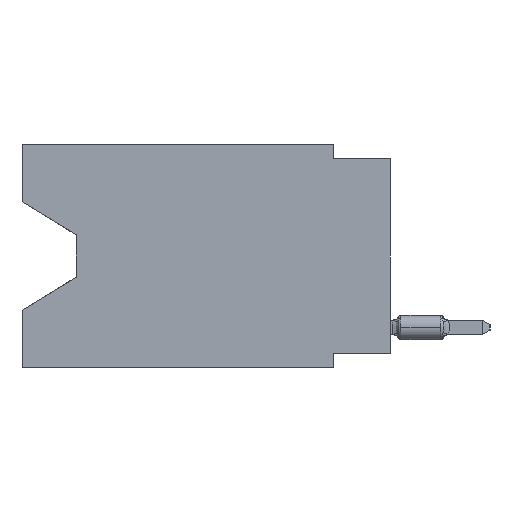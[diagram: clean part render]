
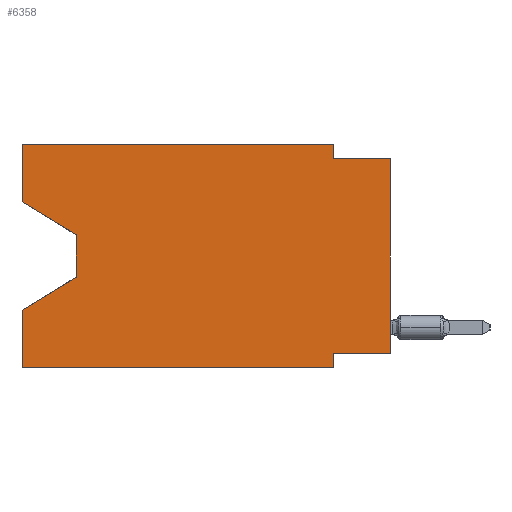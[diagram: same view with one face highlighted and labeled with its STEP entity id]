
A CAD part, left-side view. The second image highlights one B-rep face of the part: STEP entity #6358.
In plain terms, the highlighted planar face has unit normal (-1, 0, 0).
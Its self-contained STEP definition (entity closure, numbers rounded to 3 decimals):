
#1512 = VECTOR ( 'NONE', #14269, 1000. ) ;
#1819 = VERTEX_POINT ( 'NONE', #41051 ) ;
#2032 = EDGE_CURVE ( 'NONE', #39191, #20575, #32873, .T. ) ;
#2313 = LINE ( 'NONE', #47845, #11369 ) ;
#2354 = EDGE_CURVE ( 'NONE', #15973, #26219, #27699, .T. ) ;
#2417 = CARTESIAN_POINT ( 'NONE',  ( 0., 13.97, -4.013 ) ) ;
#2497 = DIRECTION ( 'NONE',  ( 0., 0., -1. ) ) ;
#3361 = EDGE_LOOP ( 'NONE', ( #6334, #10303, #36946, #3915, #14482, #22996, #16366, #15997, #44601, #26552, #22418, #24889 ) ) ;
#3915 = ORIENTED_EDGE ( 'NONE', *, *, #47639, .F. ) ;
#3995 = EDGE_CURVE ( 'NONE', #39756, #20575, #34410, .T. ) ;
#4462 = CARTESIAN_POINT ( 'NONE',  ( 0., 2.54, 0. ) ) ;
#6122 = EDGE_CURVE ( 'NONE', #18912, #26900, #34582, .T. ) ;
#6334 = ORIENTED_EDGE ( 'NONE', *, *, #33311, .T. ) ;
#6358 = ADVANCED_FACE ( 'NONE', ( #40655 ), #7126, .F. ) ;
#6839 = CARTESIAN_POINT ( 'NONE',  ( 0., 13.97, -5.893 ) ) ;
#6944 = CARTESIAN_POINT ( 'NONE',  ( 0., 0., -0.635 ) ) ;
#6964 = DIRECTION ( 'NONE',  ( 0., 0., 1. ) ) ;
#7126 = PLANE ( 'NONE',  #29096 ) ;
#7190 = LINE ( 'NONE', #6944, #41994 ) ;
#7594 = VERTEX_POINT ( 'NONE', #29432 ) ;
#10260 = EDGE_CURVE ( 'NONE', #26900, #7594, #7190, .T. ) ;
#10303 = ORIENTED_EDGE ( 'NONE', *, *, #11904, .T. ) ;
#10648 = LINE ( 'NONE', #25588, #21069 ) ;
#11043 = DIRECTION ( 'NONE',  ( 1., 0., 0. ) ) ;
#11065 = CARTESIAN_POINT ( 'NONE',  ( 0., 2.54, -0.635 ) ) ;
#11369 = VECTOR ( 'NONE', #31947, 1000. ) ;
#11904 = EDGE_CURVE ( 'NONE', #18382, #1819, #29109, .T. ) ;
#12140 = CARTESIAN_POINT ( 'NONE',  ( 0., 2.54, -9.906 ) ) ;
#12975 = DIRECTION ( 'NONE',  ( 0., 0., 1. ) ) ;
#12997 = DIRECTION ( 'NONE',  ( 0., 0., 1. ) ) ;
#13322 = DIRECTION ( 'NONE',  ( 0., -1., 0. ) ) ;
#13789 = CARTESIAN_POINT ( 'NONE',  ( 0., 13.97, -4.013 ) ) ;
#13973 = EDGE_CURVE ( 'NONE', #30000, #7594, #10648, .T. ) ;
#14126 = CARTESIAN_POINT ( 'NONE',  ( 0., 16.383, -2.546 ) ) ;
#14269 = DIRECTION ( 'NONE',  ( 0., -1., 0. ) ) ;
#14366 = DIRECTION ( 'NONE',  ( 0., -0.855, -0.519 ) ) ;
#14482 = ORIENTED_EDGE ( 'NONE', *, *, #2032, .T. ) ;
#14748 = VERTEX_POINT ( 'NONE', #17641 ) ;
#15544 = VECTOR ( 'NONE', #16872, 1000. ) ;
#15973 = VERTEX_POINT ( 'NONE', #34467 ) ;
#15997 = ORIENTED_EDGE ( 'NONE', *, *, #13973, .T. ) ;
#16366 = ORIENTED_EDGE ( 'NONE', *, *, #46910, .F. ) ;
#16872 = DIRECTION ( 'NONE',  ( 0., 0., -1. ) ) ;
#17641 = CARTESIAN_POINT ( 'NONE',  ( 0., 16.383, -7.36 ) ) ;
#18382 = VERTEX_POINT ( 'NONE', #13789 ) ;
#18912 = VERTEX_POINT ( 'NONE', #19013 ) ;
#19013 = CARTESIAN_POINT ( 'NONE',  ( 0., 2.54, 0. ) ) ;
#20175 = CARTESIAN_POINT ( 'NONE',  ( 0., 16.383, 0. ) ) ;
#20575 = VERTEX_POINT ( 'NONE', #33538 ) ;
#21069 = VECTOR ( 'NONE', #6964, 1000. ) ;
#21534 = LINE ( 'NONE', #6839, #48112 ) ;
#21873 = DIRECTION ( 'NONE',  ( 0., -1., 0. ) ) ;
#22011 = DIRECTION ( 'NONE',  ( 0., 0.855, -0.519 ) ) ;
#22083 = CARTESIAN_POINT ( 'NONE',  ( 0., 16.383, -9.906 ) ) ;
#22418 = ORIENTED_EDGE ( 'NONE', *, *, #43143, .F. ) ;
#22996 = ORIENTED_EDGE ( 'NONE', *, *, #3995, .F. ) ;
#23609 = LINE ( 'NONE', #20175, #24547 ) ;
#24547 = VECTOR ( 'NONE', #13322, 1000. ) ;
#24553 = VECTOR ( 'NONE', #14366, 1000. ) ;
#24889 = ORIENTED_EDGE ( 'NONE', *, *, #2354, .F. ) ;
#25588 = CARTESIAN_POINT ( 'NONE',  ( 0., 0., 0. ) ) ;
#26219 = VERTEX_POINT ( 'NONE', #42239 ) ;
#26552 = ORIENTED_EDGE ( 'NONE', *, *, #6122, .F. ) ;
#26900 = VERTEX_POINT ( 'NONE', #11065 ) ;
#27699 = LINE ( 'NONE', #42617, #42175 ) ;
#28408 = CARTESIAN_POINT ( 'NONE',  ( 0., 16.383, 0. ) ) ;
#29096 = AXIS2_PLACEMENT_3D ( 'NONE', #33326, #11043, #2497 ) ;
#29109 = LINE ( 'NONE', #2417, #15544 ) ;
#29396 = CARTESIAN_POINT ( 'NONE',  ( 0., 0., -9.271 ) ) ;
#29432 = CARTESIAN_POINT ( 'NONE',  ( 0., 0., -0.635 ) ) ;
#30000 = VERTEX_POINT ( 'NONE', #29396 ) ;
#31947 = DIRECTION ( 'NONE',  ( 0., 1., 0. ) ) ;
#32873 = LINE ( 'NONE', #22083, #1512 ) ;
#33311 = EDGE_CURVE ( 'NONE', #15973, #18382, #47667, .T. ) ;
#33326 = CARTESIAN_POINT ( 'NONE',  ( 0., 16.383, 0. ) ) ;
#33538 = CARTESIAN_POINT ( 'NONE',  ( 0., 2.54, -9.906 ) ) ;
#34410 = LINE ( 'NONE', #12140, #39949 ) ;
#34467 = CARTESIAN_POINT ( 'NONE',  ( 0., 16.383, -2.546 ) ) ;
#34582 = LINE ( 'NONE', #4462, #46355 ) ;
#35141 = DIRECTION ( 'NONE',  ( 0., 0., -1. ) ) ;
#36946 = ORIENTED_EDGE ( 'NONE', *, *, #46630, .T. ) ;
#39191 = VERTEX_POINT ( 'NONE', #40315 ) ;
#39722 = CARTESIAN_POINT ( 'NONE',  ( 0., 2.54, -9.271 ) ) ;
#39756 = VERTEX_POINT ( 'NONE', #39722 ) ;
#39949 = VECTOR ( 'NONE', #35141, 1000. ) ;
#40315 = CARTESIAN_POINT ( 'NONE',  ( 0., 16.383, -9.906 ) ) ;
#40655 = FACE_OUTER_BOUND ( 'NONE', #3361, .T. ) ;
#41051 = CARTESIAN_POINT ( 'NONE',  ( 0., 13.97, -5.893 ) ) ;
#41994 = VECTOR ( 'NONE', #21873, 1000. ) ;
#42175 = VECTOR ( 'NONE', #12997, 1000. ) ;
#42239 = CARTESIAN_POINT ( 'NONE',  ( 0., 16.383, 0. ) ) ;
#42617 = CARTESIAN_POINT ( 'NONE',  ( 0., 16.383, 0. ) ) ;
#43083 = LINE ( 'NONE', #28408, #43485 ) ;
#43143 = EDGE_CURVE ( 'NONE', #26219, #18912, #23609, .T. ) ;
#43485 = VECTOR ( 'NONE', #12975, 1000. ) ;
#44601 = ORIENTED_EDGE ( 'NONE', *, *, #10260, .F. ) ;
#44879 = DIRECTION ( 'NONE',  ( 0., 0., -1. ) ) ;
#46355 = VECTOR ( 'NONE', #44879, 1000. ) ;
#46630 = EDGE_CURVE ( 'NONE', #1819, #14748, #21534, .T. ) ;
#46910 = EDGE_CURVE ( 'NONE', #30000, #39756, #2313, .T. ) ;
#47639 = EDGE_CURVE ( 'NONE', #39191, #14748, #43083, .T. ) ;
#47667 = LINE ( 'NONE', #14126, #24553 ) ;
#47845 = CARTESIAN_POINT ( 'NONE',  ( 0., 0., -9.271 ) ) ;
#48112 = VECTOR ( 'NONE', #22011, 1000. ) ;
